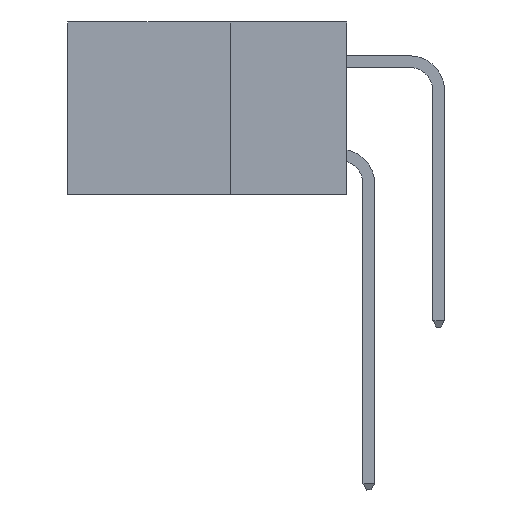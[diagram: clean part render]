
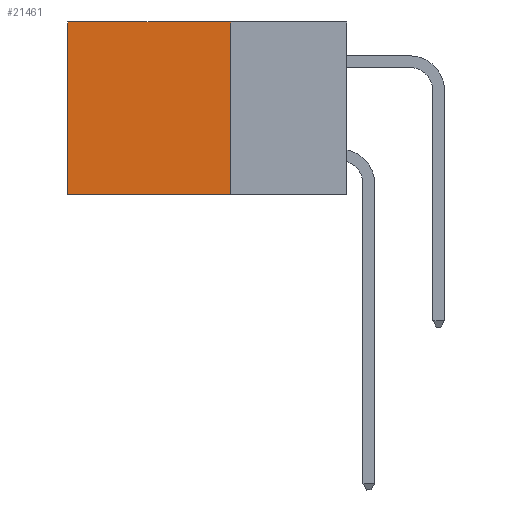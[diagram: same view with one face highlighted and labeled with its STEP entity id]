
A CAD part, left-side view. The second image highlights one B-rep face of the part: STEP entity #21461.
In plain terms, the highlighted planar face has unit normal (-1, 0, 0).
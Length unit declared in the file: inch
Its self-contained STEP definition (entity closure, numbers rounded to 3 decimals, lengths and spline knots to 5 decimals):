
#2647 = LINE ( 'NONE', #10732, #11392 ) ;
#3838 = LINE ( 'NONE', #38967, #31482 ) ;
#4066 = EDGE_CURVE ( 'NONE', #14105, #19757, #4757, .T. ) ;
#4391 = VERTEX_POINT ( 'NONE', #22640 ) ;
#4587 = DIRECTION ( 'NONE',  ( 0., 1., 0. ) ) ;
#4757 = LINE ( 'NONE', #37256, #27772 ) ;
#7488 = CARTESIAN_POINT ( 'NONE',  ( 0.2875, 0.25, 0. ) ) ;
#9063 = FACE_OUTER_BOUND ( 'NONE', #13806, .T. ) ;
#9423 = VECTOR ( 'NONE', #4587, 39.37008 ) ;
#10732 = CARTESIAN_POINT ( 'NONE',  ( 0.2875, 0.25, 0. ) ) ;
#11392 = VECTOR ( 'NONE', #20959, 39.37008 ) ;
#12708 = EDGE_CURVE ( 'NONE', #26115, #4391, #2647, .T. ) ;
#13806 = EDGE_LOOP ( 'NONE', ( #42283, #22404, #31064, #33670 ) ) ;
#13815 = PLANE ( 'NONE',  #16373 ) ;
#14105 = VERTEX_POINT ( 'NONE', #35984 ) ;
#16373 = AXIS2_PLACEMENT_3D ( 'NONE', #17099, #23049, #22901 ) ;
#17099 = CARTESIAN_POINT ( 'NONE',  ( 0.2875, 0.25, 0. ) ) ;
#19757 = VERTEX_POINT ( 'NONE', #39933 ) ;
#20603 = EDGE_CURVE ( 'NONE', #4391, #19757, #3838, .T. ) ;
#20959 = DIRECTION ( 'NONE',  ( 0., 0., -1. ) ) ;
#21461 = ADVANCED_FACE ( 'NONE', ( #9063 ), #13815, .F. ) ;
#22404 = ORIENTED_EDGE ( 'NONE', *, *, #20603, .F. ) ;
#22640 = CARTESIAN_POINT ( 'NONE',  ( 0.2875, 0.25, -0.37 ) ) ;
#22901 = DIRECTION ( 'NONE',  ( 0., 0., -1. ) ) ;
#23049 = DIRECTION ( 'NONE',  ( 1., 0., 0. ) ) ;
#26115 = VERTEX_POINT ( 'NONE', #7488 ) ;
#27772 = VECTOR ( 'NONE', #37804, 39.37008 ) ;
#28011 = CARTESIAN_POINT ( 'NONE',  ( 0.2875, 0.25, 0. ) ) ;
#29870 = EDGE_CURVE ( 'NONE', #26115, #14105, #32944, .T. ) ;
#31064 = ORIENTED_EDGE ( 'NONE', *, *, #12708, .F. ) ;
#31482 = VECTOR ( 'NONE', #41379, 39.37008 ) ;
#32944 = LINE ( 'NONE', #28011, #9423 ) ;
#33670 = ORIENTED_EDGE ( 'NONE', *, *, #29870, .T. ) ;
#35984 = CARTESIAN_POINT ( 'NONE',  ( 0.2875, 0.6, 0. ) ) ;
#37256 = CARTESIAN_POINT ( 'NONE',  ( 0.2875, 0.6, 0. ) ) ;
#37804 = DIRECTION ( 'NONE',  ( 0., 0., -1. ) ) ;
#38967 = CARTESIAN_POINT ( 'NONE',  ( 0.2875, 0.25, -0.37 ) ) ;
#39933 = CARTESIAN_POINT ( 'NONE',  ( 0.2875, 0.6, -0.37 ) ) ;
#41379 = DIRECTION ( 'NONE',  ( 0., 1., 0. ) ) ;
#42283 = ORIENTED_EDGE ( 'NONE', *, *, #4066, .T. ) ;
